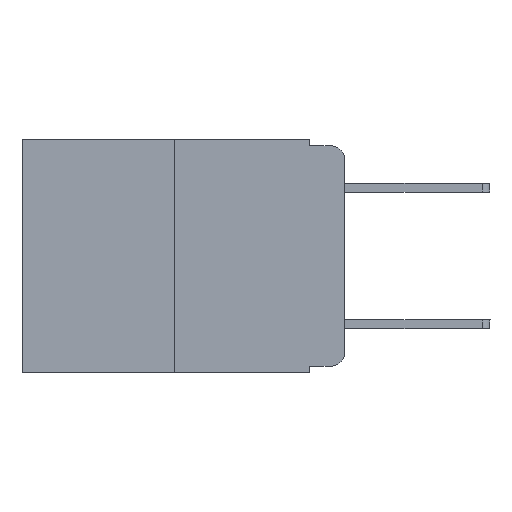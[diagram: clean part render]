
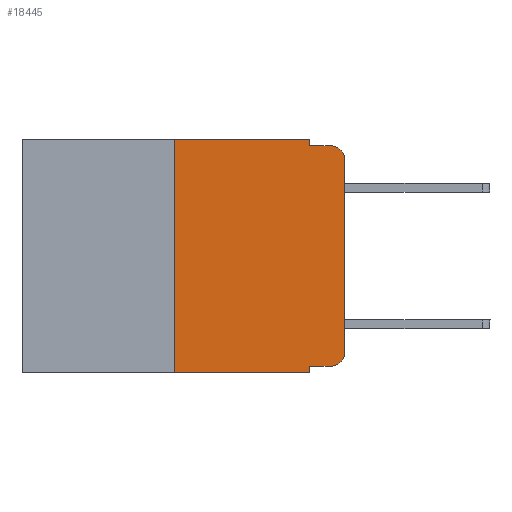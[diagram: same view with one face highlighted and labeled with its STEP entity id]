
A CAD part, left-side view. The second image highlights one B-rep face of the part: STEP entity #18445.
In plain terms, the highlighted planar face has unit normal (-1, 0, 0).
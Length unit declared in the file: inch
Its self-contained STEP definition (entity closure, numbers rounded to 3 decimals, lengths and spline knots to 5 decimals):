
#12 = VERTEX_POINT ( 'NONE', #18420 ) ;
#34 = CARTESIAN_POINT ( 'NONE',  ( 0., 0.051, 0. ) ) ;
#123 = CARTESIAN_POINT ( 'NONE',  ( 0., 0.02, -0.03 ) ) ;
#297 = VECTOR ( 'NONE', #20534, 39.37008 ) ;
#1048 = CARTESIAN_POINT ( 'NONE',  ( 0., 0.473, 0. ) ) ;
#1329 = VERTEX_POINT ( 'NONE', #13485 ) ;
#1469 = EDGE_CURVE ( 'NONE', #2555, #12, #11853, .T. ) ;
#1711 = ORIENTED_EDGE ( 'NONE', *, *, #1469, .T. ) ;
#1805 = DIRECTION ( 'NONE',  ( 0., 0., 1. ) ) ;
#1860 = ORIENTED_EDGE ( 'NONE', *, *, #14898, .T. ) ;
#2099 = VECTOR ( 'NONE', #7714, 39.37008 ) ;
#2110 = LINE ( 'NONE', #34, #19378 ) ;
#2555 = VERTEX_POINT ( 'NONE', #10182 ) ;
#2728 = DIRECTION ( 'NONE',  ( 0., 0., -1. ) ) ;
#2788 = EDGE_CURVE ( 'NONE', #1329, #16216, #13850, .T. ) ;
#2792 = ORIENTED_EDGE ( 'NONE', *, *, #14220, .F. ) ;
#2880 = CARTESIAN_POINT ( 'NONE',  ( 0., 0.02, -0.313 ) ) ;
#2903 = VERTEX_POINT ( 'NONE', #9711 ) ;
#3402 = DIRECTION ( 'NONE',  ( 0., 0., -1. ) ) ;
#3450 = FACE_OUTER_BOUND ( 'NONE', #17981, .T. ) ;
#3797 = CIRCLE ( 'NONE', #17740, 0.02 ) ;
#4022 = CARTESIAN_POINT ( 'NONE',  ( 0., 0.051, -0.01 ) ) ;
#4083 = ORIENTED_EDGE ( 'NONE', *, *, #9101, .T. ) ;
#4462 = PLANE ( 'NONE',  #15346 ) ;
#4530 = AXIS2_PLACEMENT_3D ( 'NONE', #123, #18965, #7180 ) ;
#4895 = VERTEX_POINT ( 'NONE', #5897 ) ;
#5320 = CARTESIAN_POINT ( 'NONE',  ( 0., 0.473, -0.343 ) ) ;
#5425 = EDGE_CURVE ( 'NONE', #12, #18648, #15581, .T. ) ;
#5736 = VECTOR ( 'NONE', #20676, 39.37008 ) ;
#5897 = CARTESIAN_POINT ( 'NONE',  ( 0., 0.02, -0.333 ) ) ;
#6991 = DIRECTION ( 'NONE',  ( 0., -1., 0. ) ) ;
#7154 = CARTESIAN_POINT ( 'NONE',  ( 0., 0.25, 0. ) ) ;
#7180 = DIRECTION ( 'NONE',  ( 0., 0., -1. ) ) ;
#7714 = DIRECTION ( 'NONE',  ( 0., 0., 1. ) ) ;
#7801 = EDGE_CURVE ( 'NONE', #16216, #12902, #19662, .T. ) ;
#8817 = CARTESIAN_POINT ( 'NONE',  ( 0., 0.473, 0. ) ) ;
#9101 = EDGE_CURVE ( 'NONE', #2903, #4895, #17180, .T. ) ;
#9590 = VECTOR ( 'NONE', #13194, 39.37008 ) ;
#9630 = DIRECTION ( 'NONE',  ( -1., 0., 0. ) ) ;
#9711 = CARTESIAN_POINT ( 'NONE',  ( 0., 0.051, -0.333 ) ) ;
#10182 = CARTESIAN_POINT ( 'NONE',  ( 0., 0., -0.313 ) ) ;
#10577 = ORIENTED_EDGE ( 'NONE', *, *, #10804, .T. ) ;
#10804 = EDGE_CURVE ( 'NONE', #4895, #2555, #3797, .T. ) ;
#11685 = ORIENTED_EDGE ( 'NONE', *, *, #5425, .T. ) ;
#11853 = LINE ( 'NONE', #18609, #17343 ) ;
#12183 = VECTOR ( 'NONE', #6991, 39.37008 ) ;
#12428 = VECTOR ( 'NONE', #19042, 39.37008 ) ;
#12705 = DIRECTION ( 'NONE',  ( 1., 0., 0. ) ) ;
#12902 = VERTEX_POINT ( 'NONE', #13233 ) ;
#13194 = DIRECTION ( 'NONE',  ( 0., -1., 0. ) ) ;
#13233 = CARTESIAN_POINT ( 'NONE',  ( 0., 0.051, 0. ) ) ;
#13317 = VERTEX_POINT ( 'NONE', #15159 ) ;
#13485 = CARTESIAN_POINT ( 'NONE',  ( 0., 0.25, -0.343 ) ) ;
#13850 = LINE ( 'NONE', #19501, #2099 ) ;
#13853 = LINE ( 'NONE', #4022, #5736 ) ;
#14185 = ORIENTED_EDGE ( 'NONE', *, *, #7801, .F. ) ;
#14220 = EDGE_CURVE ( 'NONE', #12902, #13317, #2110, .T. ) ;
#14898 = EDGE_CURVE ( 'NONE', #1329, #17676, #18195, .T. ) ;
#14976 = CARTESIAN_POINT ( 'NONE',  ( 0., 0.02, -0.01 ) ) ;
#15159 = CARTESIAN_POINT ( 'NONE',  ( 0., 0.051, -0.01 ) ) ;
#15346 = AXIS2_PLACEMENT_3D ( 'NONE', #1048, #12705, #2728 ) ;
#15496 = ORIENTED_EDGE ( 'NONE', *, *, #2788, .F. ) ;
#15581 = CIRCLE ( 'NONE', #4530, 0.02 ) ;
#15672 = EDGE_CURVE ( 'NONE', #2903, #17676, #21593, .T. ) ;
#15674 = CARTESIAN_POINT ( 'NONE',  ( 0., 0.051, -0.343 ) ) ;
#15676 = ORIENTED_EDGE ( 'NONE', *, *, #15672, .F. ) ;
#15816 = CARTESIAN_POINT ( 'NONE',  ( 0., 0.051, 0. ) ) ;
#15925 = ORIENTED_EDGE ( 'NONE', *, *, #19589, .F. ) ;
#16216 = VERTEX_POINT ( 'NONE', #7154 ) ;
#16841 = CARTESIAN_POINT ( 'NONE',  ( 0., 0.051, -0.333 ) ) ;
#17180 = LINE ( 'NONE', #16841, #9590 ) ;
#17343 = VECTOR ( 'NONE', #1805, 39.37008 ) ;
#17676 = VERTEX_POINT ( 'NONE', #15674 ) ;
#17740 = AXIS2_PLACEMENT_3D ( 'NONE', #2880, #9630, #19546 ) ;
#17981 = EDGE_LOOP ( 'NONE', ( #1711, #11685, #15925, #2792, #14185, #15496, #1860, #15676, #4083, #10577 ) ) ;
#18195 = LINE ( 'NONE', #5320, #12183 ) ;
#18420 = CARTESIAN_POINT ( 'NONE',  ( 0., 0., -0.03 ) ) ;
#18445 = ADVANCED_FACE ( 'NONE', ( #3450 ), #4462, .F. ) ;
#18609 = CARTESIAN_POINT ( 'NONE',  ( 0., 0., 0. ) ) ;
#18648 = VERTEX_POINT ( 'NONE', #14976 ) ;
#18965 = DIRECTION ( 'NONE',  ( -1., 0., 0. ) ) ;
#19042 = DIRECTION ( 'NONE',  ( 0., 0., -1. ) ) ;
#19378 = VECTOR ( 'NONE', #3402, 39.37008 ) ;
#19501 = CARTESIAN_POINT ( 'NONE',  ( 0., 0.25, 0. ) ) ;
#19546 = DIRECTION ( 'NONE',  ( 0., 0., -1. ) ) ;
#19589 = EDGE_CURVE ( 'NONE', #13317, #18648, #13853, .T. ) ;
#19662 = LINE ( 'NONE', #8817, #297 ) ;
#20534 = DIRECTION ( 'NONE',  ( 0., -1., 0. ) ) ;
#20676 = DIRECTION ( 'NONE',  ( 0., -1., 0. ) ) ;
#21593 = LINE ( 'NONE', #15816, #12428 ) ;
